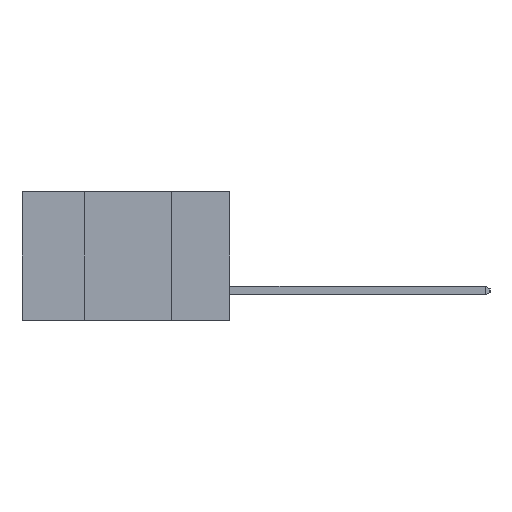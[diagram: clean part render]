
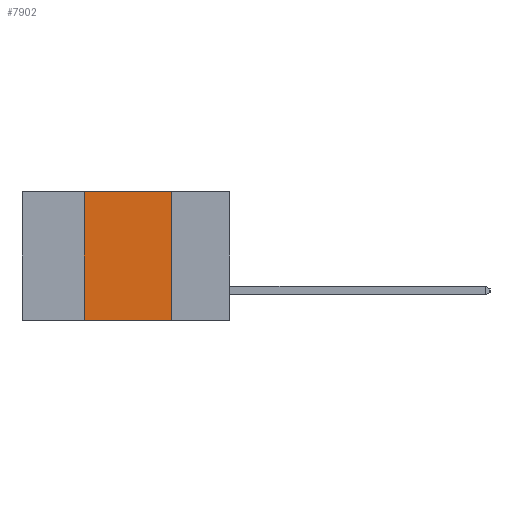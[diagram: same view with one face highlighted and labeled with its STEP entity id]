
A CAD part, left-side view. The second image highlights one B-rep face of the part: STEP entity #7902.
In plain terms, the highlighted planar face has unit normal (-1, 0, 0).
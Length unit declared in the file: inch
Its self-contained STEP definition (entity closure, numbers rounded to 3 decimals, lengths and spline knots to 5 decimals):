
#215 = CARTESIAN_POINT ( 'NONE',  ( 0., 0.17, 0. ) ) ;
#1010 = VECTOR ( 'NONE', #2880, 39.37008 ) ;
#1269 = CARTESIAN_POINT ( 'NONE',  ( 0., 0.17, -0.37 ) ) ;
#2117 = EDGE_CURVE ( 'NONE', #19017, #12428, #11966, .T. ) ;
#2807 = VECTOR ( 'NONE', #22467, 39.37008 ) ;
#2880 = DIRECTION ( 'NONE',  ( 0., -1., 0. ) ) ;
#3254 = CARTESIAN_POINT ( 'NONE',  ( 0., 0.6, 0. ) ) ;
#3272 = VERTEX_POINT ( 'NONE', #8990 ) ;
#5649 = FACE_OUTER_BOUND ( 'NONE', #9510, .T. ) ;
#7069 = EDGE_CURVE ( 'NONE', #3272, #7185, #10863, .T. ) ;
#7185 = VERTEX_POINT ( 'NONE', #215 ) ;
#7902 = ADVANCED_FACE ( 'NONE', ( #5649 ), #13865, .F. ) ;
#8023 = EDGE_CURVE ( 'NONE', #7185, #12428, #18059, .T. ) ;
#8990 = CARTESIAN_POINT ( 'NONE',  ( 0., 0.42, 0. ) ) ;
#9242 = CARTESIAN_POINT ( 'NONE',  ( 0., 0.42, -0.37 ) ) ;
#9510 = EDGE_LOOP ( 'NONE', ( #10914, #18441, #13348, #12119 ) ) ;
#10445 = DIRECTION ( 'NONE',  ( 0., 0., -1. ) ) ;
#10542 = CARTESIAN_POINT ( 'NONE',  ( 0., 0.17, -0.37 ) ) ;
#10709 = CARTESIAN_POINT ( 'NONE',  ( 0., 0.42, -0.37 ) ) ;
#10863 = LINE ( 'NONE', #3254, #1010 ) ;
#10914 = ORIENTED_EDGE ( 'NONE', *, *, #8023, .F. ) ;
#11966 = LINE ( 'NONE', #22691, #2807 ) ;
#12119 = ORIENTED_EDGE ( 'NONE', *, *, #2117, .T. ) ;
#12428 = VERTEX_POINT ( 'NONE', #1269 ) ;
#13348 = ORIENTED_EDGE ( 'NONE', *, *, #20490, .F. ) ;
#13808 = DIRECTION ( 'NONE',  ( 0., 0., -1. ) ) ;
#13844 = DIRECTION ( 'NONE',  ( 1., 0., 0. ) ) ;
#13865 = PLANE ( 'NONE',  #19689 ) ;
#14013 = CARTESIAN_POINT ( 'NONE',  ( 0., 0.6, 0. ) ) ;
#18059 = LINE ( 'NONE', #10542, #22864 ) ;
#18140 = LINE ( 'NONE', #10709, #22384 ) ;
#18441 = ORIENTED_EDGE ( 'NONE', *, *, #7069, .F. ) ;
#19017 = VERTEX_POINT ( 'NONE', #9242 ) ;
#19689 = AXIS2_PLACEMENT_3D ( 'NONE', #14013, #13844, #13808 ) ;
#20490 = EDGE_CURVE ( 'NONE', #19017, #3272, #18140, .T. ) ;
#22384 = VECTOR ( 'NONE', #23848, 39.37008 ) ;
#22467 = DIRECTION ( 'NONE',  ( 0., -1., 0. ) ) ;
#22691 = CARTESIAN_POINT ( 'NONE',  ( 0., 0.6, -0.37 ) ) ;
#22864 = VECTOR ( 'NONE', #10445, 39.37008 ) ;
#23848 = DIRECTION ( 'NONE',  ( 0., 0., 1. ) ) ;
